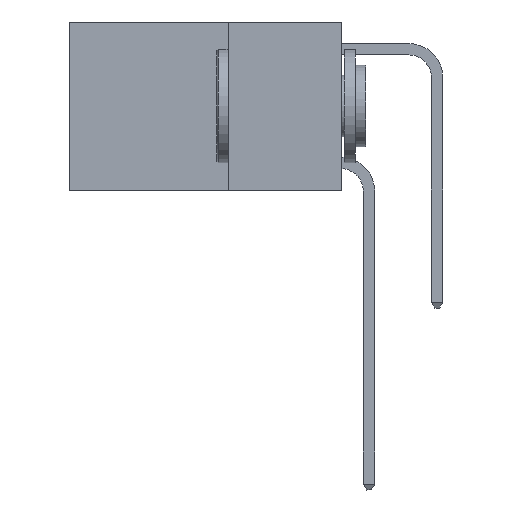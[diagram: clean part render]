
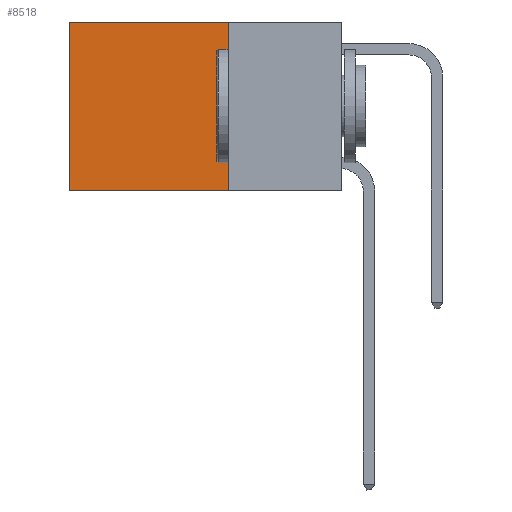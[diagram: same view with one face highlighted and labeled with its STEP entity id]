
A CAD part, left-side view. The second image highlights one B-rep face of the part: STEP entity #8518.
In plain terms, the highlighted planar face has unit normal (-1, 0, 0).
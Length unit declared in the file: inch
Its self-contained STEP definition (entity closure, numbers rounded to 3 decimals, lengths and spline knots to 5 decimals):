
#189 = VERTEX_POINT ( 'NONE', #5589 ) ;
#964 = VECTOR ( 'NONE', #3226, 39.37008 ) ;
#1143 = ORIENTED_EDGE ( 'NONE', *, *, #6510, .F. ) ;
#1241 = EDGE_CURVE ( 'NONE', #4659, #189, #8419, .T. ) ;
#1730 = DIRECTION ( 'NONE',  ( 0., 0., -1. ) ) ;
#2022 = VECTOR ( 'NONE', #6723, 39.37008 ) ;
#2151 = VECTOR ( 'NONE', #8652, 39.37008 ) ;
#2885 = ORIENTED_EDGE ( 'NONE', *, *, #1241, .F. ) ;
#3159 = VERTEX_POINT ( 'NONE', #3671 ) ;
#3226 = DIRECTION ( 'NONE',  ( 0., 1., 0. ) ) ;
#3671 = CARTESIAN_POINT ( 'NONE',  ( 0.2625, 0.25, 0. ) ) ;
#3904 = FACE_OUTER_BOUND ( 'NONE', #5754, .T. ) ;
#4659 = VERTEX_POINT ( 'NONE', #7429 ) ;
#4666 = LINE ( 'NONE', #5023, #2151 ) ;
#4671 = ORIENTED_EDGE ( 'NONE', *, *, #10146, .T. ) ;
#5023 = CARTESIAN_POINT ( 'NONE',  ( 0.2625, 0.25, 0. ) ) ;
#5336 = DIRECTION ( 'NONE',  ( 0., 0., -1. ) ) ;
#5589 = CARTESIAN_POINT ( 'NONE',  ( 0.2625, 0.6, -0.37 ) ) ;
#5653 = EDGE_CURVE ( 'NONE', #9690, #189, #8659, .T. ) ;
#5754 = EDGE_LOOP ( 'NONE', ( #10877, #2885, #1143, #4671 ) ) ;
#6280 = VECTOR ( 'NONE', #5336, 39.37008 ) ;
#6402 = CARTESIAN_POINT ( 'NONE',  ( 0.2625, 0.25, -0.37 ) ) ;
#6411 = CARTESIAN_POINT ( 'NONE',  ( 0.2625, 0.25, 0. ) ) ;
#6510 = EDGE_CURVE ( 'NONE', #3159, #4659, #9349, .T. ) ;
#6723 = DIRECTION ( 'NONE',  ( 0., 0., -1. ) ) ;
#7093 = CARTESIAN_POINT ( 'NONE',  ( 0.2625, 0.6, 0. ) ) ;
#7305 = DIRECTION ( 'NONE',  ( 1., 0., 0. ) ) ;
#7429 = CARTESIAN_POINT ( 'NONE',  ( 0.2625, 0.25, -0.37 ) ) ;
#8419 = LINE ( 'NONE', #6402, #964 ) ;
#8446 = CARTESIAN_POINT ( 'NONE',  ( 0.2625, 0.25, 0. ) ) ;
#8518 = ADVANCED_FACE ( 'NONE', ( #3904 ), #11804, .F. ) ;
#8652 = DIRECTION ( 'NONE',  ( 0., 1., 0. ) ) ;
#8659 = LINE ( 'NONE', #7093, #6280 ) ;
#9349 = LINE ( 'NONE', #8446, #2022 ) ;
#9690 = VERTEX_POINT ( 'NONE', #11641 ) ;
#10146 = EDGE_CURVE ( 'NONE', #3159, #9690, #4666, .T. ) ;
#10877 = ORIENTED_EDGE ( 'NONE', *, *, #5653, .T. ) ;
#11047 = AXIS2_PLACEMENT_3D ( 'NONE', #6411, #7305, #1730 ) ;
#11641 = CARTESIAN_POINT ( 'NONE',  ( 0.2625, 0.6, 0. ) ) ;
#11804 = PLANE ( 'NONE',  #11047 ) ;
